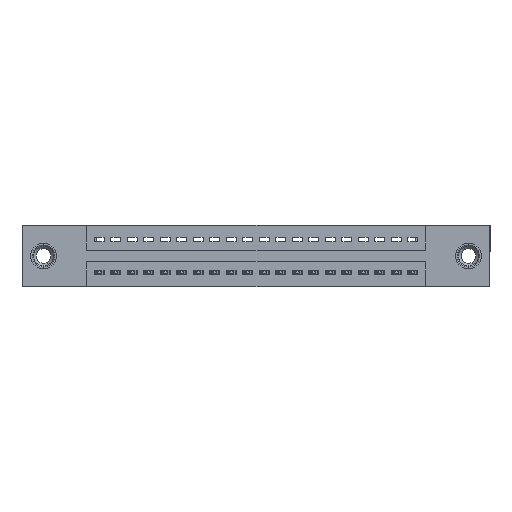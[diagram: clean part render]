
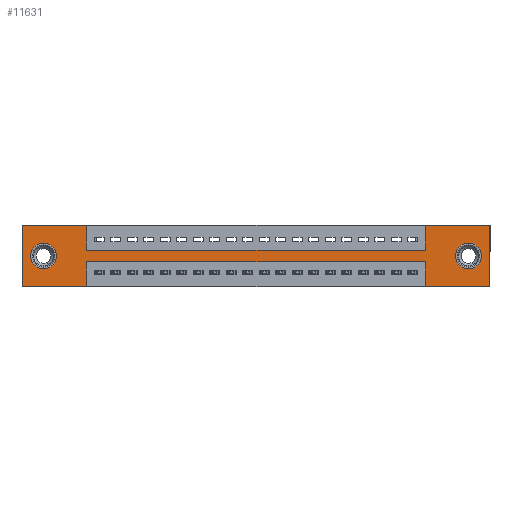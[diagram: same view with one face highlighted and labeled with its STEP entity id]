
A CAD part, front view. The second image highlights one B-rep face of the part: STEP entity #11631.
In plain terms, the highlighted planar face has unit normal (0, -1, 0).
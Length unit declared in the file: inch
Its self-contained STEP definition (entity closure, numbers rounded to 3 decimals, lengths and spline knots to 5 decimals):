
#3 = VECTOR ( 'NONE', #14781, 39.37008 ) ;
#166 = EDGE_LOOP ( 'NONE', ( #15528, #9271 ) ) ;
#287 = EDGE_CURVE ( 'NONE', #6335, #12135, #8072, .T. ) ;
#372 = PLANE ( 'NONE',  #18276 ) ;
#420 = VECTOR ( 'NONE', #726, 39.37008 ) ;
#680 = LINE ( 'NONE', #10679, #18290 ) ;
#726 = DIRECTION ( 'NONE',  ( 1., 0., 0. ) ) ;
#765 = CARTESIAN_POINT ( 'NONE',  ( 0.3925, 0., -0.15 ) ) ;
#788 = EDGE_CURVE ( 'NONE', #5327, #6997, #19776, .T. ) ;
#820 = CARTESIAN_POINT ( 'NONE',  ( 2.4425, 0., -0.22 ) ) ;
#827 = CARTESIAN_POINT ( 'NONE',  ( 0.3925, 0., -0.37 ) ) ;
#851 = DIRECTION ( 'NONE',  ( 1., 0., 0. ) ) ;
#1478 = FACE_OUTER_BOUND ( 'NONE', #18630, .T. ) ;
#1706 = DIRECTION ( 'NONE',  ( 0., 0., -1. ) ) ;
#1760 = CARTESIAN_POINT ( 'NONE',  ( 2.4425, 0., -0.15 ) ) ;
#1825 = DIRECTION ( 'NONE',  ( 0., 1., 0. ) ) ;
#2155 = CARTESIAN_POINT ( 'NONE',  ( 0.3925, 0., -0.22 ) ) ;
#2758 = EDGE_CURVE ( 'NONE', #20063, #6610, #17300, .T. ) ;
#2856 = EDGE_CURVE ( 'NONE', #12495, #19177, #680, .T. ) ;
#3112 = CARTESIAN_POINT ( 'NONE',  ( 0., 0., 0. ) ) ;
#3147 = ORIENTED_EDGE ( 'NONE', *, *, #287, .F. ) ;
#3208 = ORIENTED_EDGE ( 'NONE', *, *, #17633, .F. ) ;
#3217 = VERTEX_POINT ( 'NONE', #7514 ) ;
#3450 = CIRCLE ( 'NONE', #19326, 0.078 ) ;
#3476 = AXIS2_PLACEMENT_3D ( 'NONE', #6330, #18829, #1706 ) ;
#3686 = VERTEX_POINT ( 'NONE', #18585 ) ;
#3830 = VECTOR ( 'NONE', #8739, 39.37008 ) ;
#3852 = LINE ( 'NONE', #14362, #10889 ) ;
#3894 = LINE ( 'NONE', #3112, #5082 ) ;
#4164 = CARTESIAN_POINT ( 'NONE',  ( 0., 0., 0. ) ) ;
#4186 = DIRECTION ( 'NONE',  ( 0., 0., -1. ) ) ;
#4360 = CIRCLE ( 'NONE', #3476, 0.078 ) ;
#4639 = FACE_BOUND ( 'NONE', #16109, .T. ) ;
#4973 = CARTESIAN_POINT ( 'NONE',  ( 0., 0., -0.37 ) ) ;
#5047 = ORIENTED_EDGE ( 'NONE', *, *, #18115, .T. ) ;
#5082 = VECTOR ( 'NONE', #17139, 39.37008 ) ;
#5136 = CARTESIAN_POINT ( 'NONE',  ( 0.13, 0., -0.185 ) ) ;
#5196 = CARTESIAN_POINT ( 'NONE',  ( 0.3925, 0., -0.37 ) ) ;
#5327 = VERTEX_POINT ( 'NONE', #6831 ) ;
#5388 = LINE ( 'NONE', #12161, #19528 ) ;
#5437 = LINE ( 'NONE', #16304, #6615 ) ;
#6051 = VECTOR ( 'NONE', #9570, 39.37008 ) ;
#6330 = CARTESIAN_POINT ( 'NONE',  ( 2.705, 0., -0.185 ) ) ;
#6335 = VERTEX_POINT ( 'NONE', #17840 ) ;
#6610 = VERTEX_POINT ( 'NONE', #16194 ) ;
#6615 = VECTOR ( 'NONE', #6917, 39.37008 ) ;
#6630 = DIRECTION ( 'NONE',  ( 0., 0., 1. ) ) ;
#6697 = CARTESIAN_POINT ( 'NONE',  ( 0., 0., -0.37 ) ) ;
#6754 = CIRCLE ( 'NONE', #8398, 0.078 ) ;
#6831 = CARTESIAN_POINT ( 'NONE',  ( 2.705, 0., -0.107 ) ) ;
#6915 = EDGE_CURVE ( 'NONE', #12135, #20063, #5437, .T. ) ;
#6917 = DIRECTION ( 'NONE',  ( -1., 0., 0. ) ) ;
#6997 = VERTEX_POINT ( 'NONE', #11356 ) ;
#7319 = VERTEX_POINT ( 'NONE', #820 ) ;
#7514 = CARTESIAN_POINT ( 'NONE',  ( 2.835, 0., 0. ) ) ;
#7773 = DIRECTION ( 'NONE',  ( 0., 1., 0. ) ) ;
#8072 = LINE ( 'NONE', #827, #14672 ) ;
#8336 = EDGE_CURVE ( 'NONE', #3217, #12495, #12588, .T. ) ;
#8398 = AXIS2_PLACEMENT_3D ( 'NONE', #5136, #15872, #17358 ) ;
#8431 = CARTESIAN_POINT ( 'NONE',  ( 0.13, 0., -0.263 ) ) ;
#8515 = VERTEX_POINT ( 'NONE', #8431 ) ;
#8739 = DIRECTION ( 'NONE',  ( 0., 0., -1. ) ) ;
#8766 = FACE_BOUND ( 'NONE', #166, .T. ) ;
#9208 = DIRECTION ( 'NONE',  ( -1., 0., 0. ) ) ;
#9271 = ORIENTED_EDGE ( 'NONE', *, *, #12719, .T. ) ;
#9333 = DIRECTION ( 'NONE',  ( 0., 0., -1. ) ) ;
#9345 = ORIENTED_EDGE ( 'NONE', *, *, #6915, .F. ) ;
#9570 = DIRECTION ( 'NONE',  ( -1., 0., 0. ) ) ;
#9826 = CARTESIAN_POINT ( 'NONE',  ( 0.13, 0., -0.185 ) ) ;
#10010 = ORIENTED_EDGE ( 'NONE', *, *, #11031, .F. ) ;
#10117 = CARTESIAN_POINT ( 'NONE',  ( 0.13, 0., -0.107 ) ) ;
#10185 = ORIENTED_EDGE ( 'NONE', *, *, #16638, .F. ) ;
#10433 = LINE ( 'NONE', #18000, #14343 ) ;
#10679 = CARTESIAN_POINT ( 'NONE',  ( 0., 0., -0.37 ) ) ;
#10889 = VECTOR ( 'NONE', #16082, 39.37008 ) ;
#11031 = EDGE_CURVE ( 'NONE', #12089, #18398, #5388, .T. ) ;
#11356 = CARTESIAN_POINT ( 'NONE',  ( 2.705, 0., -0.263 ) ) ;
#11530 = DIRECTION ( 'NONE',  ( 0., 0., -1. ) ) ;
#11631 = ADVANCED_FACE ( 'NONE', ( #8766, #4639, #1478 ), #372, .T. ) ;
#11744 = EDGE_CURVE ( 'NONE', #19177, #7319, #13405, .T. ) ;
#12089 = VERTEX_POINT ( 'NONE', #1760 ) ;
#12135 = VERTEX_POINT ( 'NONE', #5196 ) ;
#12161 = CARTESIAN_POINT ( 'NONE',  ( 2.4425, 0., 0. ) ) ;
#12495 = VERTEX_POINT ( 'NONE', #14521 ) ;
#12588 = LINE ( 'NONE', #19928, #3830 ) ;
#12598 = EDGE_CURVE ( 'NONE', #6610, #3686, #17267, .T. ) ;
#12627 = VERTEX_POINT ( 'NONE', #10117 ) ;
#12719 = EDGE_CURVE ( 'NONE', #6997, #5327, #4360, .T. ) ;
#12776 = ORIENTED_EDGE ( 'NONE', *, *, #12948, .F. ) ;
#12850 = EDGE_CURVE ( 'NONE', #7319, #6335, #16533, .T. ) ;
#12948 = EDGE_CURVE ( 'NONE', #3686, #16382, #3852, .T. ) ;
#13134 = VECTOR ( 'NONE', #19829, 39.37008 ) ;
#13405 = LINE ( 'NONE', #16418, #3 ) ;
#13739 = ORIENTED_EDGE ( 'NONE', *, *, #2856, .F. ) ;
#14169 = AXIS2_PLACEMENT_3D ( 'NONE', #17119, #7773, #9333 ) ;
#14343 = VECTOR ( 'NONE', #851, 39.37008 ) ;
#14362 = CARTESIAN_POINT ( 'NONE',  ( 0.3925, 0., 0. ) ) ;
#14446 = CARTESIAN_POINT ( 'NONE',  ( 2.4425, 0., -0.37 ) ) ;
#14454 = ORIENTED_EDGE ( 'NONE', *, *, #8336, .F. ) ;
#14521 = CARTESIAN_POINT ( 'NONE',  ( 2.835, 0., -0.37 ) ) ;
#14567 = DIRECTION ( 'NONE',  ( 0., -1., 0. ) ) ;
#14672 = VECTOR ( 'NONE', #4186, 39.37008 ) ;
#14748 = ORIENTED_EDGE ( 'NONE', *, *, #11744, .F. ) ;
#14781 = DIRECTION ( 'NONE',  ( 0., 0., 1. ) ) ;
#15351 = DIRECTION ( 'NONE',  ( 0., 0., 1. ) ) ;
#15528 = ORIENTED_EDGE ( 'NONE', *, *, #788, .T. ) ;
#15574 = EDGE_CURVE ( 'NONE', #8515, #12627, #3450, .T. ) ;
#15872 = DIRECTION ( 'NONE',  ( 0., 1., 0. ) ) ;
#15920 = ORIENTED_EDGE ( 'NONE', *, *, #12850, .F. ) ;
#16082 = DIRECTION ( 'NONE',  ( 0., 0., -1. ) ) ;
#16109 = EDGE_LOOP ( 'NONE', ( #5047, #19884 ) ) ;
#16194 = CARTESIAN_POINT ( 'NONE',  ( 0., 0., 0. ) ) ;
#16304 = CARTESIAN_POINT ( 'NONE',  ( 0., 0., -0.37 ) ) ;
#16345 = CARTESIAN_POINT ( 'NONE',  ( 2.4425, 0., 0. ) ) ;
#16382 = VERTEX_POINT ( 'NONE', #765 ) ;
#16418 = CARTESIAN_POINT ( 'NONE',  ( 2.4425, 0., -0.37 ) ) ;
#16533 = LINE ( 'NONE', #2155, #6051 ) ;
#16638 = EDGE_CURVE ( 'NONE', #18398, #3217, #3894, .T. ) ;
#16748 = ORIENTED_EDGE ( 'NONE', *, *, #12598, .F. ) ;
#17119 = CARTESIAN_POINT ( 'NONE',  ( 2.705, 0., -0.185 ) ) ;
#17139 = DIRECTION ( 'NONE',  ( 1., 0., 0. ) ) ;
#17267 = LINE ( 'NONE', #19404, #420 ) ;
#17300 = LINE ( 'NONE', #4164, #13134 ) ;
#17358 = DIRECTION ( 'NONE',  ( 0., 0., 1. ) ) ;
#17633 = EDGE_CURVE ( 'NONE', #16382, #12089, #10433, .T. ) ;
#17840 = CARTESIAN_POINT ( 'NONE',  ( 0.3925, 0., -0.22 ) ) ;
#18000 = CARTESIAN_POINT ( 'NONE',  ( 0.3925, 0., -0.15 ) ) ;
#18115 = EDGE_CURVE ( 'NONE', #12627, #8515, #6754, .T. ) ;
#18276 = AXIS2_PLACEMENT_3D ( 'NONE', #6697, #14567, #11530 ) ;
#18290 = VECTOR ( 'NONE', #9208, 39.37008 ) ;
#18398 = VERTEX_POINT ( 'NONE', #16345 ) ;
#18585 = CARTESIAN_POINT ( 'NONE',  ( 0.3925, 0., 0. ) ) ;
#18630 = EDGE_LOOP ( 'NONE', ( #3147, #15920, #14748, #13739, #14454, #10185, #10010, #3208, #12776, #16748, #18672, #9345 ) ) ;
#18672 = ORIENTED_EDGE ( 'NONE', *, *, #2758, .F. ) ;
#18829 = DIRECTION ( 'NONE',  ( 0., 1., 0. ) ) ;
#19177 = VERTEX_POINT ( 'NONE', #14446 ) ;
#19326 = AXIS2_PLACEMENT_3D ( 'NONE', #9826, #1825, #6630 ) ;
#19404 = CARTESIAN_POINT ( 'NONE',  ( 0., 0., 0. ) ) ;
#19528 = VECTOR ( 'NONE', #15351, 39.37008 ) ;
#19776 = CIRCLE ( 'NONE', #14169, 0.078 ) ;
#19829 = DIRECTION ( 'NONE',  ( 0., 0., 1. ) ) ;
#19884 = ORIENTED_EDGE ( 'NONE', *, *, #15574, .T. ) ;
#19928 = CARTESIAN_POINT ( 'NONE',  ( 2.835, 0., 0. ) ) ;
#20063 = VERTEX_POINT ( 'NONE', #4973 ) ;
